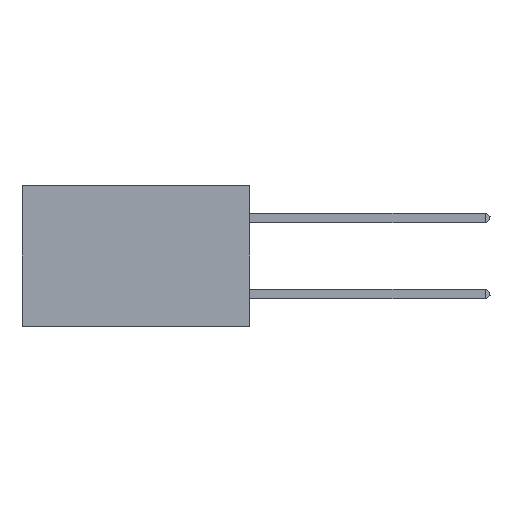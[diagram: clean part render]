
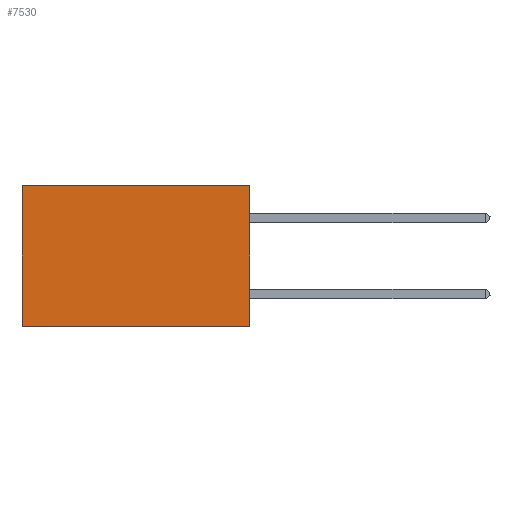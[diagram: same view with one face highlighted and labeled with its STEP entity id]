
A CAD part, left-side view. The second image highlights one B-rep face of the part: STEP entity #7530.
In plain terms, the highlighted planar face has unit normal (-1, 0, 0).
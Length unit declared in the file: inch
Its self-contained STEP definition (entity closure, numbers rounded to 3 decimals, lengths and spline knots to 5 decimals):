
#1523 = DIRECTION ( 'NONE',  ( 0., 0., -1. ) ) ;
#1788 = ORIENTED_EDGE ( 'NONE', *, *, #15665, .F. ) ;
#1997 = EDGE_CURVE ( 'NONE', #20486, #19530, #19804, .T. ) ;
#2222 = VECTOR ( 'NONE', #9390, 39.37008 ) ;
#3248 = LINE ( 'NONE', #18916, #2222 ) ;
#4270 = CARTESIAN_POINT ( 'NONE',  ( 0.2875, 0.6, 0. ) ) ;
#4281 = VECTOR ( 'NONE', #11301, 39.37008 ) ;
#4466 = VECTOR ( 'NONE', #5791, 39.37008 ) ;
#5535 = ORIENTED_EDGE ( 'NONE', *, *, #13177, .T. ) ;
#5762 = VERTEX_POINT ( 'NONE', #17406 ) ;
#5791 = DIRECTION ( 'NONE',  ( 0., 1., 0. ) ) ;
#6403 = EDGE_CURVE ( 'NONE', #20180, #5762, #3248, .T. ) ;
#7530 = ADVANCED_FACE ( 'NONE', ( #10534 ), #17149, .F. ) ;
#7605 = DIRECTION ( 'NONE',  ( 1., 0., 0. ) ) ;
#9042 = ORIENTED_EDGE ( 'NONE', *, *, #6403, .F. ) ;
#9197 = LINE ( 'NONE', #12889, #4281 ) ;
#9369 = LINE ( 'NONE', #13834, #4466 ) ;
#9390 = DIRECTION ( 'NONE',  ( 0., 0., -1. ) ) ;
#10009 = CARTESIAN_POINT ( 'NONE',  ( 0.2875, 0.6, 0. ) ) ;
#10388 = AXIS2_PLACEMENT_3D ( 'NONE', #15562, #7605, #18747 ) ;
#10534 = FACE_OUTER_BOUND ( 'NONE', #19293, .T. ) ;
#11301 = DIRECTION ( 'NONE',  ( 0., 1., 0. ) ) ;
#12158 = ORIENTED_EDGE ( 'NONE', *, *, #1997, .T. ) ;
#12889 = CARTESIAN_POINT ( 'NONE',  ( 0.2875, 0., -0.37 ) ) ;
#13177 = EDGE_CURVE ( 'NONE', #20180, #20486, #9369, .T. ) ;
#13834 = CARTESIAN_POINT ( 'NONE',  ( 0.2875, 0., 0. ) ) ;
#14984 = CARTESIAN_POINT ( 'NONE',  ( 0.2875, 0., 0. ) ) ;
#15562 = CARTESIAN_POINT ( 'NONE',  ( 0.2875, 0., 0. ) ) ;
#15665 = EDGE_CURVE ( 'NONE', #5762, #19530, #9197, .T. ) ;
#16119 = VECTOR ( 'NONE', #1523, 39.37008 ) ;
#17149 = PLANE ( 'NONE',  #10388 ) ;
#17406 = CARTESIAN_POINT ( 'NONE',  ( 0.2875, 0., -0.37 ) ) ;
#18747 = DIRECTION ( 'NONE',  ( 0., 0., -1. ) ) ;
#18916 = CARTESIAN_POINT ( 'NONE',  ( 0.2875, 0., 0. ) ) ;
#19293 = EDGE_LOOP ( 'NONE', ( #12158, #1788, #9042, #5535 ) ) ;
#19375 = CARTESIAN_POINT ( 'NONE',  ( 0.2875, 0.6, -0.37 ) ) ;
#19530 = VERTEX_POINT ( 'NONE', #19375 ) ;
#19804 = LINE ( 'NONE', #10009, #16119 ) ;
#20180 = VERTEX_POINT ( 'NONE', #14984 ) ;
#20486 = VERTEX_POINT ( 'NONE', #4270 ) ;
